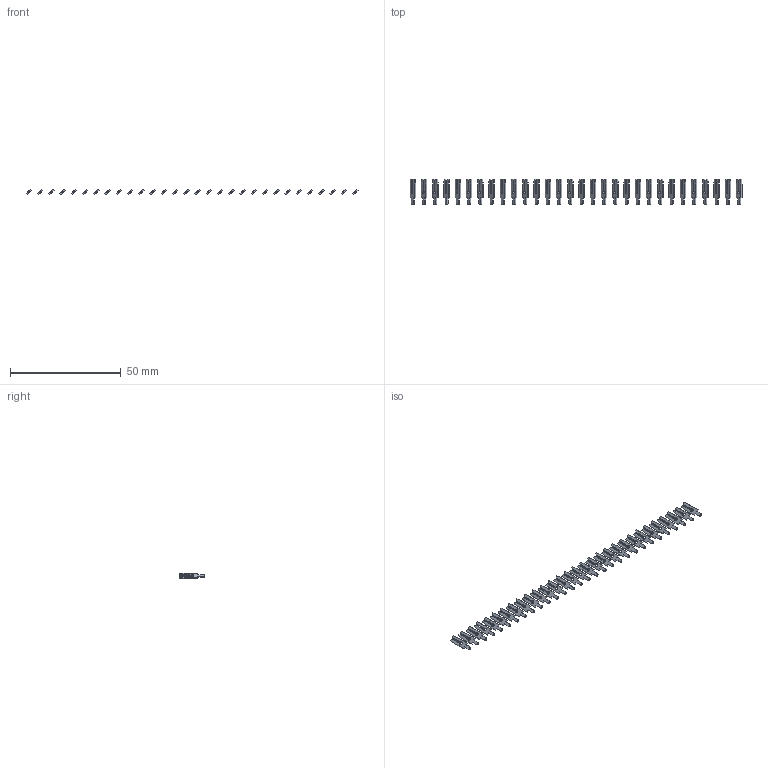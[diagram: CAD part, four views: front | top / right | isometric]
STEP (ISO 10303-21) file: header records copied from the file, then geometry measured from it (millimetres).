
FILE_DESCRIPTION (( 'STEP AP203' ), '1' );
FILE_NAME ('106-030-250-200.STEP', '2020-04-16T19:30:31', ( '' ), ( '' ), 'SwSTEP 2.0', 'SolidWorks 2016', '' );
FILE_SCHEMA (( 'CONFIG_CONTROL_DESIGN' ));
Length unit declared in the file: inch
Products named in the file (2): 100-290-001_100-290-250; 106-030-250-200
Assembly tree (30 placements, depth 2):
  106-030-250-200
    100-290-001_100-290-250  x30
Bounding box: 149.85 x 11.48 x 2.53 mm (x, y, z)
Volume: 468.1 mm3; surface area: 2200.5 mm2
Topology: 30 solids, 30 shells, 720 faces, 1980 edges, 1320 vertices
Faces by surface type: plane 600, cylinder 120
Entity records: 1886 total; most frequent: DIRECTION 184, CARTESIAN_POINT 179, ORIENTED_EDGE 132, COORDINATED_UNIVERSAL_TIME_OFFSET 70, LOCAL_TIME 70, DATE_AND_TIME 70, CALENDAR_DATE 70, EDGE_CURVE 66
